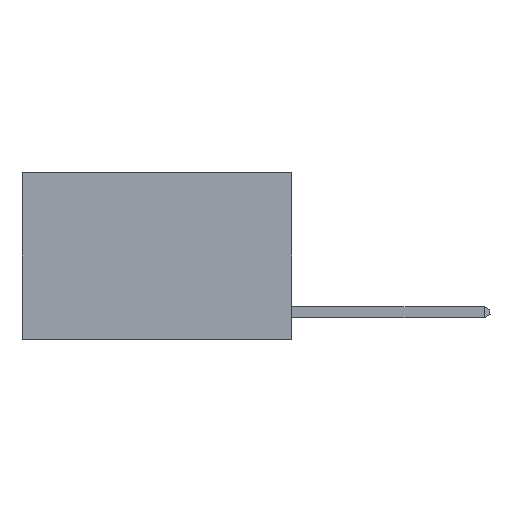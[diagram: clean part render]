
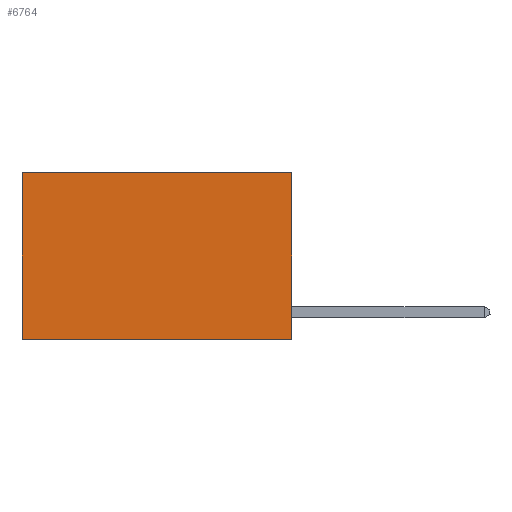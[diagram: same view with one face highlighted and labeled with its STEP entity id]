
A CAD part, left-side view. The second image highlights one B-rep face of the part: STEP entity #6764.
In plain terms, the highlighted planar face has unit normal (-1, 0, 0).
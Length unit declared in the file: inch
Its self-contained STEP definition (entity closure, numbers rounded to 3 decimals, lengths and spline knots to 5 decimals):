
#432 = AXIS2_PLACEMENT_3D ( 'NONE', #14175, #1781, #11442 ) ;
#933 = VECTOR ( 'NONE', #14885, 39.37008 ) ;
#1274 = VECTOR ( 'NONE', #3922, 39.37008 ) ;
#1781 = DIRECTION ( 'NONE',  ( 1., 0., 0. ) ) ;
#2047 = CARTESIAN_POINT ( 'NONE',  ( 0.2625, 0., 0. ) ) ;
#2545 = CARTESIAN_POINT ( 'NONE',  ( 0.2625, 0.6, 0. ) ) ;
#2766 = ORIENTED_EDGE ( 'NONE', *, *, #4301, .T. ) ;
#3922 = DIRECTION ( 'NONE',  ( 0., 0., -1. ) ) ;
#4301 = EDGE_CURVE ( 'NONE', #17422, #8391, #8144, .T. ) ;
#4612 = CARTESIAN_POINT ( 'NONE',  ( 0.2625, 0., -0.37 ) ) ;
#4751 = CARTESIAN_POINT ( 'NONE',  ( 0.2625, 0., 0. ) ) ;
#5179 = FACE_OUTER_BOUND ( 'NONE', #14416, .T. ) ;
#5349 = VERTEX_POINT ( 'NONE', #4612 ) ;
#5371 = VECTOR ( 'NONE', #6072, 39.37008 ) ;
#6072 = DIRECTION ( 'NONE',  ( 0., 1., 0. ) ) ;
#6227 = VECTOR ( 'NONE', #13121, 39.37008 ) ;
#6764 = ADVANCED_FACE ( 'NONE', ( #5179 ), #10008, .F. ) ;
#6876 = ORIENTED_EDGE ( 'NONE', *, *, #8130, .F. ) ;
#7307 = ORIENTED_EDGE ( 'NONE', *, *, #17560, .T. ) ;
#8130 = EDGE_CURVE ( 'NONE', #5349, #8391, #16471, .T. ) ;
#8144 = LINE ( 'NONE', #2545, #1274 ) ;
#8391 = VERTEX_POINT ( 'NONE', #13453 ) ;
#8917 = CARTESIAN_POINT ( 'NONE',  ( 0.2625, 0.6, 0. ) ) ;
#9056 = EDGE_CURVE ( 'NONE', #10351, #5349, #13589, .T. ) ;
#10008 = PLANE ( 'NONE',  #432 ) ;
#10351 = VERTEX_POINT ( 'NONE', #2047 ) ;
#11442 = DIRECTION ( 'NONE',  ( 0., 0., -1. ) ) ;
#11588 = CARTESIAN_POINT ( 'NONE',  ( 0.2625, 0., -0.37 ) ) ;
#13121 = DIRECTION ( 'NONE',  ( 0., 0., -1. ) ) ;
#13453 = CARTESIAN_POINT ( 'NONE',  ( 0.2625, 0.6, -0.37 ) ) ;
#13458 = CARTESIAN_POINT ( 'NONE',  ( 0.2625, 0., 0. ) ) ;
#13589 = LINE ( 'NONE', #4751, #6227 ) ;
#14175 = CARTESIAN_POINT ( 'NONE',  ( 0.2625, 0., 0. ) ) ;
#14273 = ORIENTED_EDGE ( 'NONE', *, *, #9056, .F. ) ;
#14416 = EDGE_LOOP ( 'NONE', ( #2766, #6876, #14273, #7307 ) ) ;
#14885 = DIRECTION ( 'NONE',  ( 0., 1., 0. ) ) ;
#15687 = LINE ( 'NONE', #13458, #933 ) ;
#16471 = LINE ( 'NONE', #11588, #5371 ) ;
#17422 = VERTEX_POINT ( 'NONE', #8917 ) ;
#17560 = EDGE_CURVE ( 'NONE', #10351, #17422, #15687, .T. ) ;
